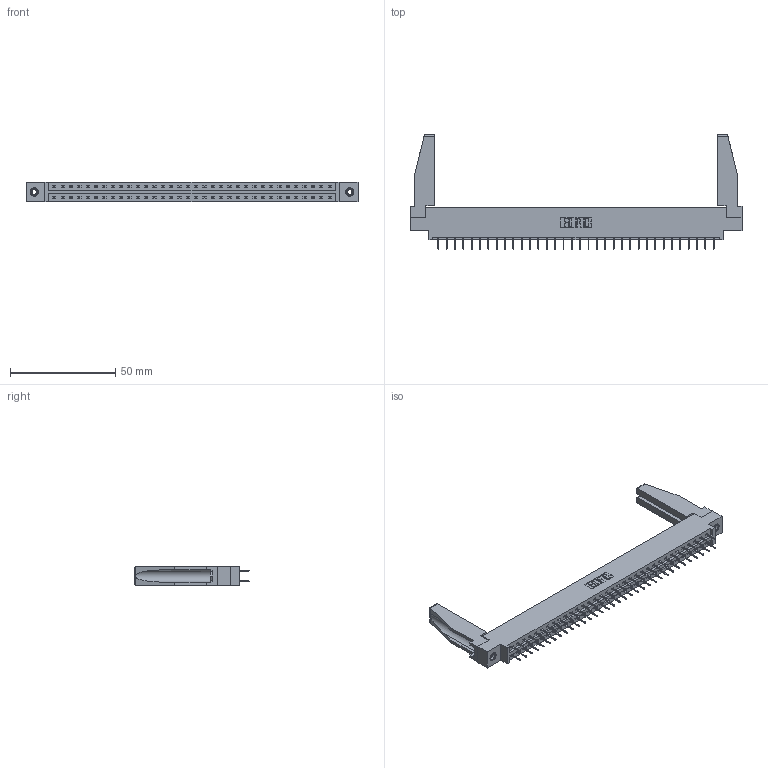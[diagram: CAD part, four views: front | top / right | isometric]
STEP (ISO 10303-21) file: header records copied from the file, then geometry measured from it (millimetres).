
FILE_DESCRIPTION (( 'STEP AP203' ), '1' );
FILE_NAME ('387-068-524-878.STEP', '2019-10-19T20:47:16', ( '' ), ( '' ), 'SwSTEP 2.0', 'SolidWorks 2016', '' );
FILE_SCHEMA (( 'CONFIG_CONTROL_DESIGN' ));
Length unit declared in the file: inch
Products named in the file (5): 387-068-524-878; 307-220-078; 345-292-001_345-293-124; 337 Part_0.170 Offset - 0.156 Dia-TI; 345-250-001_345-250-001-102
Assembly tree (73 placements, depth 2):
  387-068-524-878
    337 Part_0.170 Offset - 0.156 Dia-TI
    345-292-001_345-293-124  x68
    345-250-001_345-250-001-102  x2
    307-220-078  x2
Bounding box: 157.73 x 54.49 x 9.4 mm (x, y, z)
Volume: 20289.7 mm3; surface area: 21964.9 mm2
Topology: 73 solids, 73 shells, 4192 faces, 11873 edges, 7634 vertices
Faces by surface type: plane 3150, cylinder 1026, cone 12, torus 4
Entity records: 30042 total; most frequent: CARTESIAN_POINT 5068, ORIENTED_EDGE 4960, DIRECTION 4332, EDGE_CURVE 2480, LINE 2318, VECTOR 2318, VERTEX_POINT 1644, AXIS2_PLACEMENT_3D 1007
